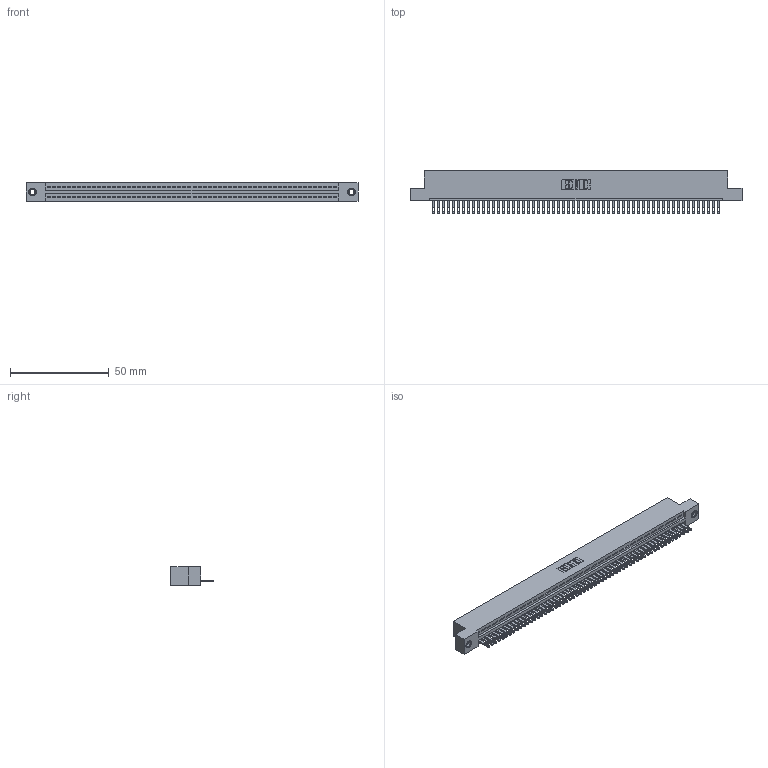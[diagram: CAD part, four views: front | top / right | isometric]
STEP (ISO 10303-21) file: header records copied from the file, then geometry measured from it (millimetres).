
FILE_DESCRIPTION (( 'STEP AP203' ), '1' );
FILE_NAME ('345-058-500-107.STEP', '2019-10-10T15:10:47', ( '' ), ( '' ), 'SwSTEP 2.0', 'SolidWorks 2016', '' );
FILE_SCHEMA (( 'CONFIG_CONTROL_DESIGN' ));
Length unit declared in the file: inch
Products named in the file (4): 345-292-001_345-293-100; 345-058-500-107; 345-250-001_345-250-005-103; 345 Part_Flush Mounting Lugs - 0.156 Dia-TI
Assembly tree (61 placements, depth 2):
  345-058-500-107
    345 Part_Flush Mounting Lugs - 0.156 Dia-TI
    345-292-001_345-293-100  x58
    345-250-001_345-250-005-103  x2
Bounding box: 168.53 x 21.51 x 9.4 mm (x, y, z)
Volume: 16160.5 mm3; surface area: 21856.1 mm2
Topology: 61 solids, 61 shells, 3318 faces, 10221 edges, 6806 vertices
Faces by surface type: plane 2084, cylinder 1218, cone 12, torus 4
Entity records: 42614 total; most frequent: CARTESIAN_POINT 7361, ORIENTED_EDGE 7346, DIRECTION 6435, EDGE_CURVE 3673, VECTOR 3285, LINE 3285, VERTEX_POINT 2444, AXIS2_PLACEMENT_3D 1575
